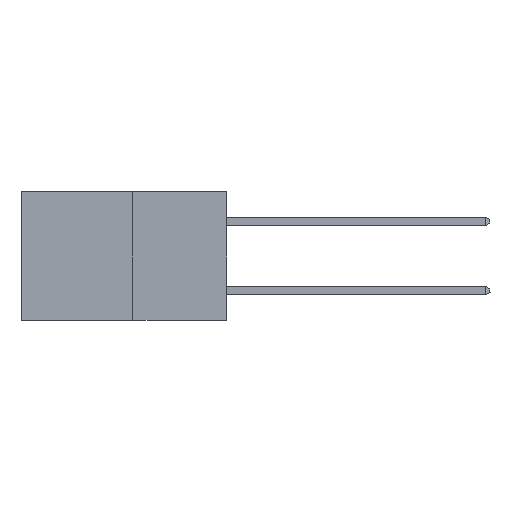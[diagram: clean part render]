
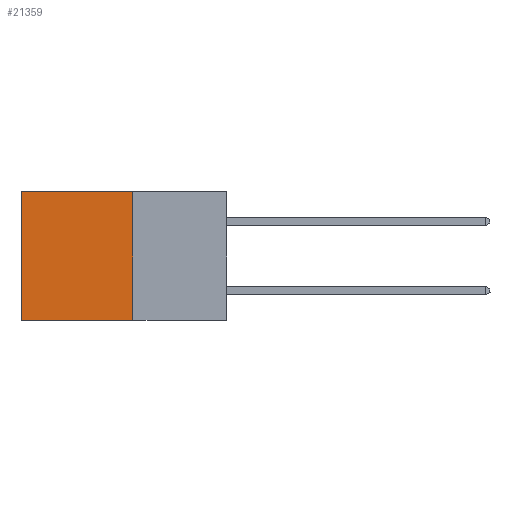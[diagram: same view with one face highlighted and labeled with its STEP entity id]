
A CAD part, left-side view. The second image highlights one B-rep face of the part: STEP entity #21359.
In plain terms, the highlighted planar face has unit normal (-1, 0, 0).
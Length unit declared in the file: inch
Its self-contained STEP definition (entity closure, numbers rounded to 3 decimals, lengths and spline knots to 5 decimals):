
#71 = EDGE_CURVE ( 'NONE', #15622, #1291, #5728, .T. ) ;
#386 = VECTOR ( 'NONE', #20044, 39.37008 ) ;
#805 = DIRECTION ( 'NONE',  ( 0., 0., -1. ) ) ;
#1015 = LINE ( 'NONE', #16479, #10576 ) ;
#1019 = VERTEX_POINT ( 'NONE', #22911 ) ;
#1291 = VERTEX_POINT ( 'NONE', #16758 ) ;
#1746 = VERTEX_POINT ( 'NONE', #14741 ) ;
#1818 = PLANE ( 'NONE',  #21916 ) ;
#4415 = CARTESIAN_POINT ( 'NONE',  ( 0.277, 0.27, -0.37 ) ) ;
#4461 = LINE ( 'NONE', #22042, #18087 ) ;
#4706 = FACE_OUTER_BOUND ( 'NONE', #8137, .T. ) ;
#5416 = DIRECTION ( 'NONE',  ( 0., 0., -1. ) ) ;
#5703 = EDGE_CURVE ( 'NONE', #1746, #1019, #10462, .T. ) ;
#5728 = LINE ( 'NONE', #4415, #386 ) ;
#6983 = EDGE_CURVE ( 'NONE', #1019, #1291, #1015, .T. ) ;
#8137 = EDGE_LOOP ( 'NONE', ( #19069, #10375, #11545, #21952 ) ) ;
#10375 = ORIENTED_EDGE ( 'NONE', *, *, #71, .F. ) ;
#10462 = LINE ( 'NONE', #14454, #20343 ) ;
#10576 = VECTOR ( 'NONE', #16462, 39.37008 ) ;
#11545 = ORIENTED_EDGE ( 'NONE', *, *, #18422, .F. ) ;
#14306 = CARTESIAN_POINT ( 'NONE',  ( 0.277, 0.27, -0.37 ) ) ;
#14430 = DIRECTION ( 'NONE',  ( 0., 1., 0. ) ) ;
#14454 = CARTESIAN_POINT ( 'NONE',  ( 0.277, 0.27, 0. ) ) ;
#14741 = CARTESIAN_POINT ( 'NONE',  ( 0.277, 0.27, 0. ) ) ;
#15622 = VERTEX_POINT ( 'NONE', #19850 ) ;
#16078 = DIRECTION ( 'NONE',  ( 1., 0., 0. ) ) ;
#16462 = DIRECTION ( 'NONE',  ( 0., 0., -1. ) ) ;
#16479 = CARTESIAN_POINT ( 'NONE',  ( 0.277, 0.59, -0.37 ) ) ;
#16758 = CARTESIAN_POINT ( 'NONE',  ( 0.277, 0.59, -0.37 ) ) ;
#18087 = VECTOR ( 'NONE', #805, 39.37008 ) ;
#18422 = EDGE_CURVE ( 'NONE', #1746, #15622, #4461, .T. ) ;
#19069 = ORIENTED_EDGE ( 'NONE', *, *, #6983, .T. ) ;
#19850 = CARTESIAN_POINT ( 'NONE',  ( 0.277, 0.27, -0.37 ) ) ;
#20044 = DIRECTION ( 'NONE',  ( 0., 1., 0. ) ) ;
#20343 = VECTOR ( 'NONE', #14430, 39.37008 ) ;
#21359 = ADVANCED_FACE ( 'NONE', ( #4706 ), #1818, .F. ) ;
#21916 = AXIS2_PLACEMENT_3D ( 'NONE', #14306, #16078, #5416 ) ;
#21952 = ORIENTED_EDGE ( 'NONE', *, *, #5703, .T. ) ;
#22042 = CARTESIAN_POINT ( 'NONE',  ( 0.277, 0.27, -0.37 ) ) ;
#22911 = CARTESIAN_POINT ( 'NONE',  ( 0.277, 0.59, 0. ) ) ;
